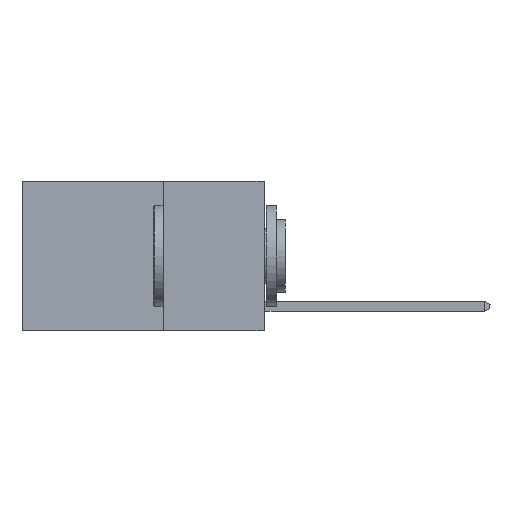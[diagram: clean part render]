
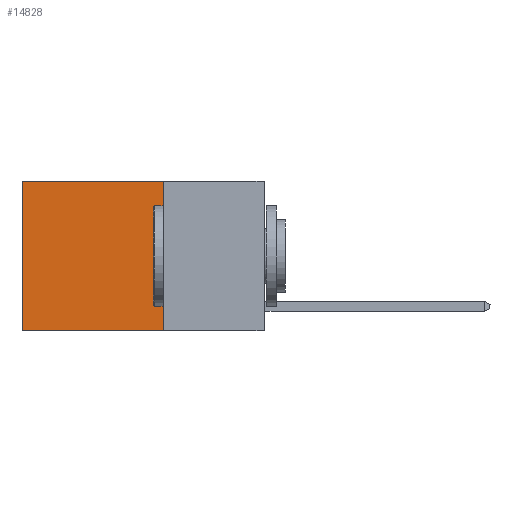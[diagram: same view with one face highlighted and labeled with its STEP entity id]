
A CAD part, left-side view. The second image highlights one B-rep face of the part: STEP entity #14828.
In plain terms, the highlighted planar face has unit normal (-1, 0, 0).
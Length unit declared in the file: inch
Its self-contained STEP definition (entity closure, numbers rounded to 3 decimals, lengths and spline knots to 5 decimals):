
#63 = DIRECTION ( 'NONE',  ( 0., 1., 0. ) ) ;
#1356 = EDGE_CURVE ( 'NONE', #15500, #8370, #6202, .T. ) ;
#1475 = CARTESIAN_POINT ( 'NONE',  ( 0.2625, 0.25, 0. ) ) ;
#1813 = LINE ( 'NONE', #4613, #6082 ) ;
#2378 = CARTESIAN_POINT ( 'NONE',  ( 0.2625, 0.6, -0.37 ) ) ;
#2680 = ORIENTED_EDGE ( 'NONE', *, *, #4273, .F. ) ;
#2742 = PLANE ( 'NONE',  #18364 ) ;
#3781 = CARTESIAN_POINT ( 'NONE',  ( 0.2625, 0.25, -0.37 ) ) ;
#3908 = CARTESIAN_POINT ( 'NONE',  ( 0.2625, 0.6, 0. ) ) ;
#4236 = EDGE_LOOP ( 'NONE', ( #17635, #2680, #7426, #5982 ) ) ;
#4273 = EDGE_CURVE ( 'NONE', #8370, #5003, #8044, .T. ) ;
#4613 = CARTESIAN_POINT ( 'NONE',  ( 0.2625, 0.6, 0. ) ) ;
#4717 = CARTESIAN_POINT ( 'NONE',  ( 0.2625, 0.25, -0.37 ) ) ;
#5003 = VERTEX_POINT ( 'NONE', #2378 ) ;
#5982 = ORIENTED_EDGE ( 'NONE', *, *, #12500, .T. ) ;
#6082 = VECTOR ( 'NONE', #19026, 39.37008 ) ;
#6202 = LINE ( 'NONE', #12473, #8258 ) ;
#6628 = VERTEX_POINT ( 'NONE', #3908 ) ;
#7318 = DIRECTION ( 'NONE',  ( 0., 0., -1. ) ) ;
#7426 = ORIENTED_EDGE ( 'NONE', *, *, #1356, .F. ) ;
#8044 = LINE ( 'NONE', #4717, #13080 ) ;
#8258 = VECTOR ( 'NONE', #18760, 39.37008 ) ;
#8370 = VERTEX_POINT ( 'NONE', #3781 ) ;
#8949 = EDGE_CURVE ( 'NONE', #6628, #5003, #1813, .T. ) ;
#9055 = CARTESIAN_POINT ( 'NONE',  ( 0.2625, 0.25, 0. ) ) ;
#9537 = LINE ( 'NONE', #1475, #18625 ) ;
#11187 = DIRECTION ( 'NONE',  ( 0., 1., 0. ) ) ;
#12473 = CARTESIAN_POINT ( 'NONE',  ( 0.2625, 0.25, 0. ) ) ;
#12500 = EDGE_CURVE ( 'NONE', #15500, #6628, #9537, .T. ) ;
#12696 = CARTESIAN_POINT ( 'NONE',  ( 0.2625, 0.25, 0. ) ) ;
#13080 = VECTOR ( 'NONE', #63, 39.37008 ) ;
#14828 = ADVANCED_FACE ( 'NONE', ( #16977 ), #2742, .F. ) ;
#15500 = VERTEX_POINT ( 'NONE', #12696 ) ;
#16977 = FACE_OUTER_BOUND ( 'NONE', #4236, .T. ) ;
#17635 = ORIENTED_EDGE ( 'NONE', *, *, #8949, .T. ) ;
#18364 = AXIS2_PLACEMENT_3D ( 'NONE', #9055, #18419, #7318 ) ;
#18419 = DIRECTION ( 'NONE',  ( 1., 0., 0. ) ) ;
#18625 = VECTOR ( 'NONE', #11187, 39.37008 ) ;
#18760 = DIRECTION ( 'NONE',  ( 0., 0., -1. ) ) ;
#19026 = DIRECTION ( 'NONE',  ( 0., 0., -1. ) ) ;
